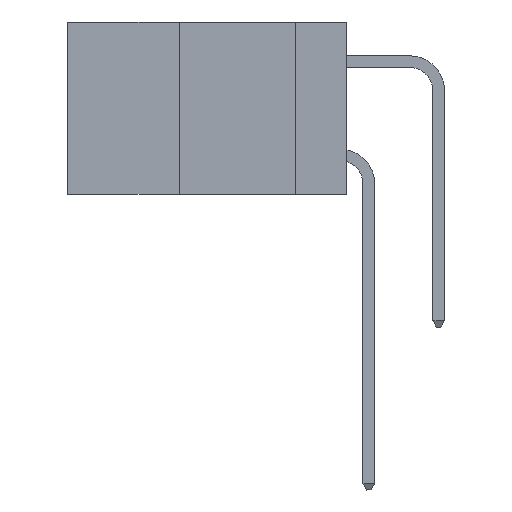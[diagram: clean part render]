
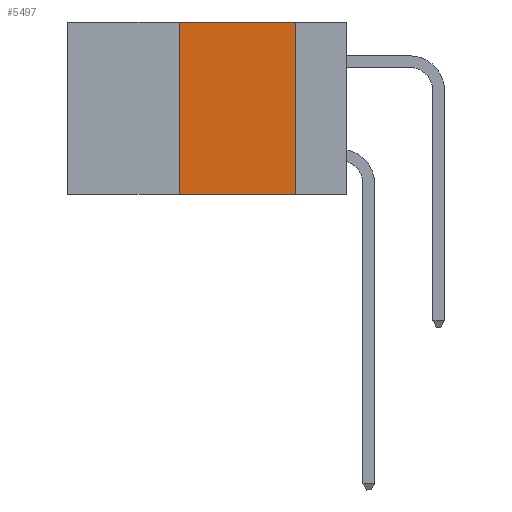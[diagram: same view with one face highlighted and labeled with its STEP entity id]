
A CAD part, left-side view. The second image highlights one B-rep face of the part: STEP entity #5497.
In plain terms, the highlighted planar face has unit normal (-1, 0, 0).
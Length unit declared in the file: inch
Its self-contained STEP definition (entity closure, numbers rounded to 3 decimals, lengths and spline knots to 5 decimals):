
#166 = VERTEX_POINT ( 'NONE', #15187 ) ;
#239 = VERTEX_POINT ( 'NONE', #12116 ) ;
#292 = CARTESIAN_POINT ( 'NONE',  ( 0., 0.6, 0. ) ) ;
#463 = LINE ( 'NONE', #11388, #8194 ) ;
#790 = VECTOR ( 'NONE', #12817, 39.37008 ) ;
#912 = DIRECTION ( 'NONE',  ( 0., -1., 0. ) ) ;
#1252 = EDGE_CURVE ( 'NONE', #15094, #16167, #15634, .T. ) ;
#1595 = DIRECTION ( 'NONE',  ( 0., -1., 0. ) ) ;
#2538 = ORIENTED_EDGE ( 'NONE', *, *, #4967, .T. ) ;
#2617 = EDGE_CURVE ( 'NONE', #166, #15094, #463, .T. ) ;
#4967 = EDGE_CURVE ( 'NONE', #166, #239, #11493, .T. ) ;
#5130 = DIRECTION ( 'NONE',  ( 0., 0., 1. ) ) ;
#5277 = EDGE_CURVE ( 'NONE', #16167, #239, #12697, .T. ) ;
#5310 = FACE_OUTER_BOUND ( 'NONE', #11222, .T. ) ;
#5497 = ADVANCED_FACE ( 'NONE', ( #5310 ), #11300, .F. ) ;
#6273 = CARTESIAN_POINT ( 'NONE',  ( 0., 0.36, 0. ) ) ;
#7028 = CARTESIAN_POINT ( 'NONE',  ( 0., 0.6, -0.37 ) ) ;
#8194 = VECTOR ( 'NONE', #5130, 39.37008 ) ;
#9190 = DIRECTION ( 'NONE',  ( 1., 0., 0. ) ) ;
#11222 = EDGE_LOOP ( 'NONE', ( #12789, #15968, #11846, #2538 ) ) ;
#11300 = PLANE ( 'NONE',  #13304 ) ;
#11360 = CARTESIAN_POINT ( 'NONE',  ( 0., 0.6, 0. ) ) ;
#11388 = CARTESIAN_POINT ( 'NONE',  ( 0., 0.36, 0. ) ) ;
#11493 = LINE ( 'NONE', #7028, #12331 ) ;
#11846 = ORIENTED_EDGE ( 'NONE', *, *, #2617, .F. ) ;
#12116 = CARTESIAN_POINT ( 'NONE',  ( 0., 0.11, -0.37 ) ) ;
#12214 = VECTOR ( 'NONE', #1595, 39.37008 ) ;
#12331 = VECTOR ( 'NONE', #912, 39.37008 ) ;
#12507 = CARTESIAN_POINT ( 'NONE',  ( 0., 0.11, 0. ) ) ;
#12697 = LINE ( 'NONE', #12931, #790 ) ;
#12789 = ORIENTED_EDGE ( 'NONE', *, *, #5277, .F. ) ;
#12817 = DIRECTION ( 'NONE',  ( 0., 0., -1. ) ) ;
#12931 = CARTESIAN_POINT ( 'NONE',  ( 0., 0.11, 0. ) ) ;
#13304 = AXIS2_PLACEMENT_3D ( 'NONE', #11360, #9190, #14205 ) ;
#14205 = DIRECTION ( 'NONE',  ( 0., 0., -1. ) ) ;
#15094 = VERTEX_POINT ( 'NONE', #6273 ) ;
#15187 = CARTESIAN_POINT ( 'NONE',  ( 0., 0.36, -0.37 ) ) ;
#15634 = LINE ( 'NONE', #292, #12214 ) ;
#15968 = ORIENTED_EDGE ( 'NONE', *, *, #1252, .F. ) ;
#16167 = VERTEX_POINT ( 'NONE', #12507 ) ;
